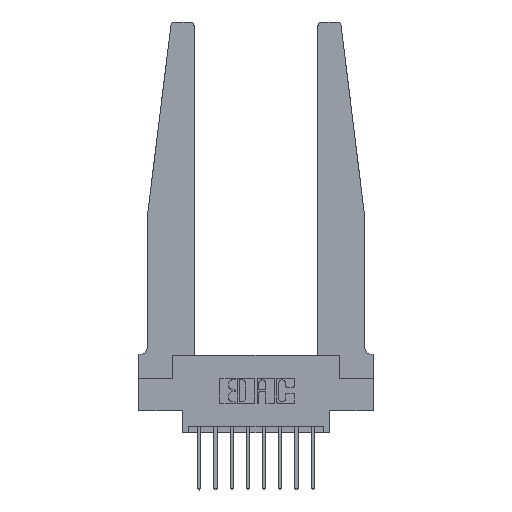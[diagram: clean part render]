
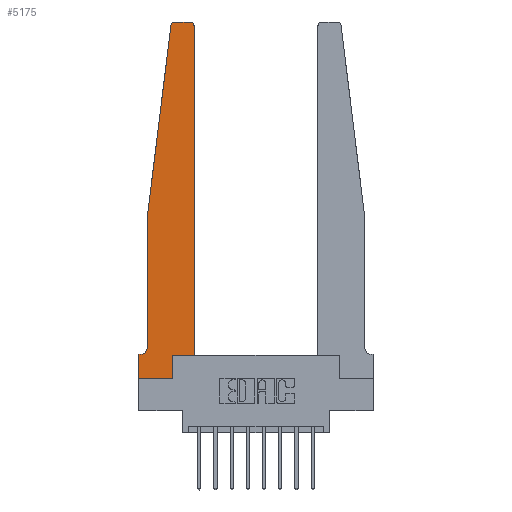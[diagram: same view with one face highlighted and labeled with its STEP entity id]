
A CAD part, top view. The second image highlights one B-rep face of the part: STEP entity #5175.
In plain terms, the highlighted planar face has unit normal (0, 0, 1).
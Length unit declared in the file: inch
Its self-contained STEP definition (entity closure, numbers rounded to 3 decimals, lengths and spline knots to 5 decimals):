
#150 = ORIENTED_EDGE ( 'NONE', *, *, #13654, .T. ) ;
#157 = CARTESIAN_POINT ( 'NONE',  ( 0.425, 2.72, 0.37 ) ) ;
#240 = CARTESIAN_POINT ( 'NONE',  ( 0.425, 0.18, 0.37 ) ) ;
#516 = ORIENTED_EDGE ( 'NONE', *, *, #6299, .T. ) ;
#1059 = CARTESIAN_POINT ( 'NONE',  ( 0.2605, 0.18, 0.37 ) ) ;
#1132 = LINE ( 'NONE', #3750, #12873 ) ;
#1218 = EDGE_LOOP ( 'NONE', ( #2847, #14369, #6865, #9302, #5813, #516, #7914, #150, #3741, #6727, #9965, #12876 ) ) ;
#1221 = VECTOR ( 'NONE', #9668, 39.37008 ) ;
#1362 = DIRECTION ( 'NONE',  ( 1., 0., 0. ) ) ;
#1720 = CARTESIAN_POINT ( 'NONE',  ( 0.015, 0.2375, 0.37 ) ) ;
#1895 = CARTESIAN_POINT ( 'NONE',  ( 0., 0.1875, 0.37 ) ) ;
#2003 = CARTESIAN_POINT ( 'NONE',  ( 0., 0., 0.37 ) ) ;
#2267 = CARTESIAN_POINT ( 'NONE',  ( 0.27653, 2.72, 0.37 ) ) ;
#2302 = DIRECTION ( 'NONE',  ( -0.122, -0.992, 0. ) ) ;
#2366 = DIRECTION ( 'NONE',  ( 0., -1., 0. ) ) ;
#2389 = VECTOR ( 'NONE', #2366, 39.37008 ) ;
#2402 = AXIS2_PLACEMENT_3D ( 'NONE', #14615, #3250, #11232 ) ;
#2514 = AXIS2_PLACEMENT_3D ( 'NONE', #2267, #10243, #3418 ) ;
#2534 = EDGE_CURVE ( 'NONE', #5033, #9234, #12846, .T. ) ;
#2847 = ORIENTED_EDGE ( 'NONE', *, *, #7956, .T. ) ;
#2855 = DIRECTION ( 'NONE',  ( -1., 0., 0. ) ) ;
#2997 = CARTESIAN_POINT ( 'NONE',  ( 0.065, 1.25, 0.37 ) ) ;
#3133 = CARTESIAN_POINT ( 'NONE',  ( 0.395, 2.72, 0.37 ) ) ;
#3139 = VERTEX_POINT ( 'NONE', #5084 ) ;
#3250 = DIRECTION ( 'NONE',  ( 0., 0., 1. ) ) ;
#3262 = CARTESIAN_POINT ( 'NONE',  ( 0.395, 2.75, 0.37 ) ) ;
#3418 = DIRECTION ( 'NONE',  ( 1., 0., 0. ) ) ;
#3509 = VECTOR ( 'NONE', #6206, 39.37008 ) ;
#3582 = VERTEX_POINT ( 'NONE', #13842 ) ;
#3741 = ORIENTED_EDGE ( 'NONE', *, *, #13467, .T. ) ;
#3750 = CARTESIAN_POINT ( 'NONE',  ( 0.25, 2.75, 0.37 ) ) ;
#3807 = VECTOR ( 'NONE', #7555, 39.37008 ) ;
#4252 = LINE ( 'NONE', #7392, #1221 ) ;
#4279 = DIRECTION ( 'NONE',  ( 1., 0., 0. ) ) ;
#4313 = CARTESIAN_POINT ( 'NONE',  ( 0.24675, 2.72367, 0.37 ) ) ;
#4376 = VERTEX_POINT ( 'NONE', #9674 ) ;
#4636 = CARTESIAN_POINT ( 'NONE',  ( 0., 0., 0.37 ) ) ;
#5033 = VERTEX_POINT ( 'NONE', #2997 ) ;
#5084 = CARTESIAN_POINT ( 'NONE',  ( 0.27653, 2.75, 0.37 ) ) ;
#5156 = LINE ( 'NONE', #240, #10843 ) ;
#5175 = ADVANCED_FACE ( 'NONE', ( #8300 ), #6626, .T. ) ;
#5675 = VERTEX_POINT ( 'NONE', #1895 ) ;
#5813 = ORIENTED_EDGE ( 'NONE', *, *, #9844, .T. ) ;
#5926 = VERTEX_POINT ( 'NONE', #6863 ) ;
#5964 = EDGE_CURVE ( 'NONE', #5675, #5926, #10762, .T. ) ;
#6206 = DIRECTION ( 'NONE',  ( 0., 1., 0. ) ) ;
#6271 = AXIS2_PLACEMENT_3D ( 'NONE', #1720, #9678, #2855 ) ;
#6299 = EDGE_CURVE ( 'NONE', #3582, #5675, #6842, .T. ) ;
#6626 = PLANE ( 'NONE',  #2402 ) ;
#6727 = ORIENTED_EDGE ( 'NONE', *, *, #11886, .T. ) ;
#6842 = LINE ( 'NONE', #14380, #3807 ) ;
#6863 = CARTESIAN_POINT ( 'NONE',  ( 0., 0., 0.37 ) ) ;
#6865 = ORIENTED_EDGE ( 'NONE', *, *, #13185, .T. ) ;
#7292 = CIRCLE ( 'NONE', #2514, 0.03 ) ;
#7392 = CARTESIAN_POINT ( 'NONE',  ( 0.2605, 0.18, 0.37 ) ) ;
#7555 = DIRECTION ( 'NONE',  ( -1., 0., 0. ) ) ;
#7804 = VECTOR ( 'NONE', #14565, 39.37008 ) ;
#7914 = ORIENTED_EDGE ( 'NONE', *, *, #5964, .T. ) ;
#7956 = EDGE_CURVE ( 'NONE', #11669, #3139, #1132, .T. ) ;
#8300 = FACE_OUTER_BOUND ( 'NONE', #1218, .T. ) ;
#9234 = VERTEX_POINT ( 'NONE', #14393 ) ;
#9302 = ORIENTED_EDGE ( 'NONE', *, *, #2534, .T. ) ;
#9375 = CARTESIAN_POINT ( 'NONE',  ( 0.065, 1.25, 0.37 ) ) ;
#9668 = DIRECTION ( 'NONE',  ( 0., 1., 0. ) ) ;
#9674 = CARTESIAN_POINT ( 'NONE',  ( 0.2605, 0., 0.37 ) ) ;
#9678 = DIRECTION ( 'NONE',  ( 0., 0., -1. ) ) ;
#9681 = AXIS2_PLACEMENT_3D ( 'NONE', #3133, #11107, #4279 ) ;
#9844 = EDGE_CURVE ( 'NONE', #9234, #3582, #12299, .T. ) ;
#9941 = LINE ( 'NONE', #11917, #3509 ) ;
#9965 = ORIENTED_EDGE ( 'NONE', *, *, #14001, .T. ) ;
#10052 = VERTEX_POINT ( 'NONE', #4313 ) ;
#10243 = DIRECTION ( 'NONE',  ( 0., 0., 1. ) ) ;
#10282 = CARTESIAN_POINT ( 'NONE',  ( 0.065, 1.25, 0.37 ) ) ;
#10392 = VERTEX_POINT ( 'NONE', #1059 ) ;
#10516 = DIRECTION ( 'NONE',  ( 0., -1., 0. ) ) ;
#10762 = LINE ( 'NONE', #4636, #2389 ) ;
#10822 = LINE ( 'NONE', #2003, #7804 ) ;
#10832 = LINE ( 'NONE', #10282, #14229 ) ;
#10843 = VECTOR ( 'NONE', #1362, 39.37008 ) ;
#11107 = DIRECTION ( 'NONE',  ( 0., 0., 1. ) ) ;
#11232 = DIRECTION ( 'NONE',  ( 1., 0., 0. ) ) ;
#11669 = VERTEX_POINT ( 'NONE', #3262 ) ;
#11738 = DIRECTION ( 'NONE',  ( -1., 0., 0. ) ) ;
#11886 = EDGE_CURVE ( 'NONE', #10392, #13970, #5156, .T. ) ;
#11917 = CARTESIAN_POINT ( 'NONE',  ( 0.425, 0.18, 0.37 ) ) ;
#12299 = CIRCLE ( 'NONE', #6271, 0.05 ) ;
#12469 = CIRCLE ( 'NONE', #9681, 0.03 ) ;
#12505 = VECTOR ( 'NONE', #10516, 39.37008 ) ;
#12797 = EDGE_CURVE ( 'NONE', #13225, #11669, #12469, .T. ) ;
#12846 = LINE ( 'NONE', #9375, #12505 ) ;
#12873 = VECTOR ( 'NONE', #11738, 39.37008 ) ;
#12876 = ORIENTED_EDGE ( 'NONE', *, *, #12797, .T. ) ;
#12976 = EDGE_CURVE ( 'NONE', #3139, #10052, #7292, .T. ) ;
#12997 = CARTESIAN_POINT ( 'NONE',  ( 0.425, 0.18, 0.37 ) ) ;
#13185 = EDGE_CURVE ( 'NONE', #10052, #5033, #10832, .T. ) ;
#13225 = VERTEX_POINT ( 'NONE', #157 ) ;
#13467 = EDGE_CURVE ( 'NONE', #4376, #10392, #4252, .T. ) ;
#13654 = EDGE_CURVE ( 'NONE', #5926, #4376, #10822, .T. ) ;
#13842 = CARTESIAN_POINT ( 'NONE',  ( 0.015, 0.1875, 0.37 ) ) ;
#13970 = VERTEX_POINT ( 'NONE', #12997 ) ;
#14001 = EDGE_CURVE ( 'NONE', #13970, #13225, #9941, .T. ) ;
#14229 = VECTOR ( 'NONE', #2302, 39.37008 ) ;
#14369 = ORIENTED_EDGE ( 'NONE', *, *, #12976, .T. ) ;
#14380 = CARTESIAN_POINT ( 'NONE',  ( 0.065, 0.1875, 0.37 ) ) ;
#14393 = CARTESIAN_POINT ( 'NONE',  ( 0.065, 0.2375, 0.37 ) ) ;
#14565 = DIRECTION ( 'NONE',  ( 1., 0., 0. ) ) ;
#14615 = CARTESIAN_POINT ( 'NONE',  ( 0., 0.1875, 0.37 ) ) ;
